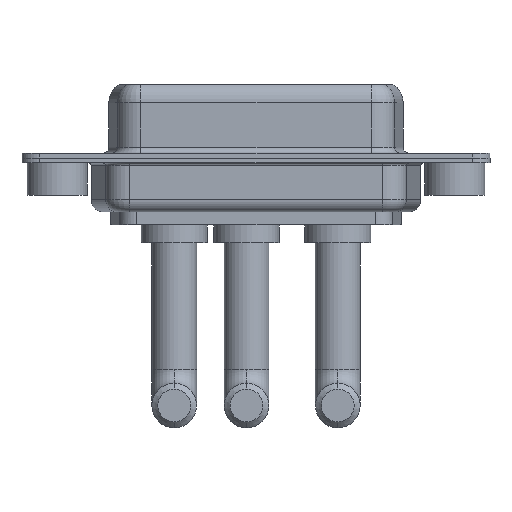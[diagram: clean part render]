
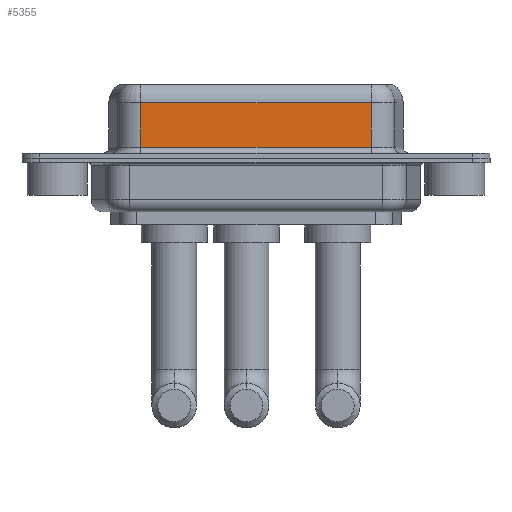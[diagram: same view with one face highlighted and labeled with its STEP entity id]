
A CAD part, front view. The second image highlights one B-rep face of the part: STEP entity #5355.
In plain terms, the highlighted planar face has unit normal (0, -1, 0).
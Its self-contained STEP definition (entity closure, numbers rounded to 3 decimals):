
#99 = LINE ( 'NONE', #9357, #10226 ) ;
#124 = VERTEX_POINT ( 'NONE', #3646 ) ;
#293 = EDGE_CURVE ( 'NONE', #124, #1584, #9216, .T. ) ;
#652 = PLANE ( 'NONE',  #10610 ) ;
#722 = DIRECTION ( 'NONE',  ( 0., 0., -1. ) ) ;
#785 = LINE ( 'NONE', #13452, #11252 ) ;
#1391 = EDGE_LOOP ( 'NONE', ( #13082, #11340, #10257, #9516 ) ) ;
#1583 = CARTESIAN_POINT ( 'NONE',  ( 26.287, -3.95, 0.9 ) ) ;
#1584 = VERTEX_POINT ( 'NONE', #1583 ) ;
#2376 = VERTEX_POINT ( 'NONE', #5120 ) ;
#3646 = CARTESIAN_POINT ( 'NONE',  ( 26.287, -3.95, 4.65 ) ) ;
#3790 = CARTESIAN_POINT ( 'NONE',  ( 26.287, -3.95, 6.4 ) ) ;
#4047 = EDGE_CURVE ( 'NONE', #2376, #9217, #785, .T. ) ;
#5120 = CARTESIAN_POINT ( 'NONE',  ( 7.013, -3.95, 4.65 ) ) ;
#5355 = ADVANCED_FACE ( 'NONE', ( #11243 ), #652, .F. ) ;
#5791 = CARTESIAN_POINT ( 'NONE',  ( 7.013, -3.95, 0.9 ) ) ;
#6857 = LINE ( 'NONE', #13298, #11787 ) ;
#9216 = LINE ( 'NONE', #13450, #13153 ) ;
#9217 = VERTEX_POINT ( 'NONE', #5791 ) ;
#9357 = CARTESIAN_POINT ( 'NONE',  ( 26.287, -3.95, 0.9 ) ) ;
#9516 = ORIENTED_EDGE ( 'NONE', *, *, #13673, .T. ) ;
#10226 = VECTOR ( 'NONE', #11587, 1000. ) ;
#10257 = ORIENTED_EDGE ( 'NONE', *, *, #4047, .T. ) ;
#10331 = DIRECTION ( 'NONE',  ( 0., 1., 0. ) ) ;
#10610 = AXIS2_PLACEMENT_3D ( 'NONE', #3790, #10331, #13387 ) ;
#11016 = DIRECTION ( 'NONE',  ( -1., 0., 0. ) ) ;
#11165 = DIRECTION ( 'NONE',  ( 0., 0., -1. ) ) ;
#11243 = FACE_OUTER_BOUND ( 'NONE', #1391, .T. ) ;
#11252 = VECTOR ( 'NONE', #722, 1000. ) ;
#11340 = ORIENTED_EDGE ( 'NONE', *, *, #12689, .T. ) ;
#11587 = DIRECTION ( 'NONE',  ( 1., 0., 0. ) ) ;
#11787 = VECTOR ( 'NONE', #11016, 1000. ) ;
#12689 = EDGE_CURVE ( 'NONE', #124, #2376, #6857, .T. ) ;
#13082 = ORIENTED_EDGE ( 'NONE', *, *, #293, .F. ) ;
#13153 = VECTOR ( 'NONE', #11165, 1000. ) ;
#13298 = CARTESIAN_POINT ( 'NONE',  ( 26.287, -3.95, 4.65 ) ) ;
#13387 = DIRECTION ( 'NONE',  ( 0., 0., 1. ) ) ;
#13450 = CARTESIAN_POINT ( 'NONE',  ( 26.287, -3.95, 6.4 ) ) ;
#13452 = CARTESIAN_POINT ( 'NONE',  ( 7.013, -3.95, 6.4 ) ) ;
#13673 = EDGE_CURVE ( 'NONE', #9217, #1584, #99, .T. ) ;
